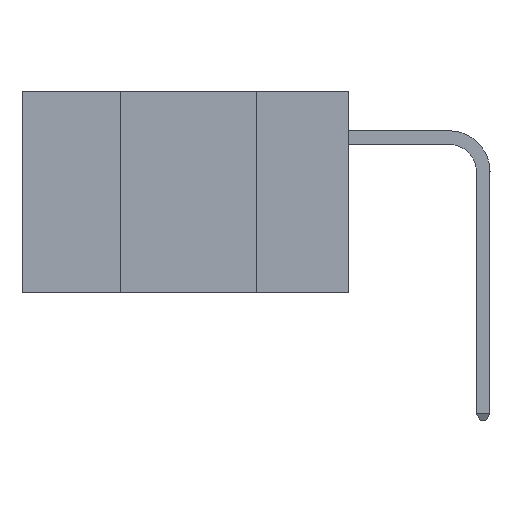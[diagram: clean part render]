
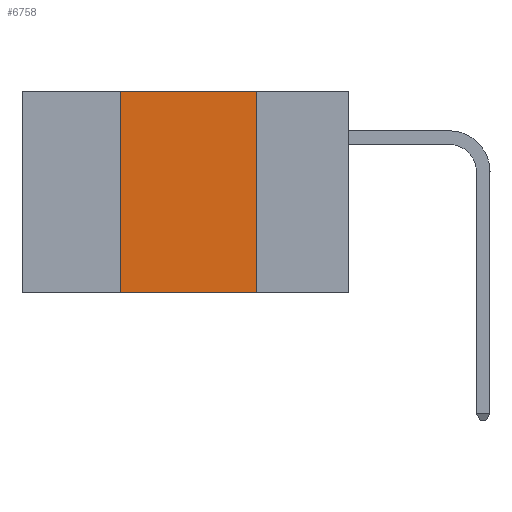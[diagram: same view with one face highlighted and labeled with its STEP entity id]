
A CAD part, left-side view. The second image highlights one B-rep face of the part: STEP entity #6758.
In plain terms, the highlighted planar face has unit normal (-1, 0, 0).
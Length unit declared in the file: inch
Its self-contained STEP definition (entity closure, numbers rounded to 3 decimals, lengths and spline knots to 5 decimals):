
#599 = DIRECTION ( 'NONE',  ( 1., 0., 0. ) ) ;
#921 = CARTESIAN_POINT ( 'NONE',  ( 0., 0.17, -0.37 ) ) ;
#3271 = ORIENTED_EDGE ( 'NONE', *, *, #20356, .F. ) ;
#4081 = DIRECTION ( 'NONE',  ( 0., -1., 0. ) ) ;
#4486 = CARTESIAN_POINT ( 'NONE',  ( 0., 0.17, 0. ) ) ;
#4714 = CARTESIAN_POINT ( 'NONE',  ( 0., 0.6, 0. ) ) ;
#6479 = EDGE_CURVE ( 'NONE', #21021, #20581, #16606, .T. ) ;
#6677 = CARTESIAN_POINT ( 'NONE',  ( 0., 0.42, 0. ) ) ;
#6758 = ADVANCED_FACE ( 'NONE', ( #10083 ), #6932, .F. ) ;
#6932 = PLANE ( 'NONE',  #14544 ) ;
#7320 = VECTOR ( 'NONE', #18434, 39.37008 ) ;
#8654 = CARTESIAN_POINT ( 'NONE',  ( 0., 0.6, 0. ) ) ;
#8744 = ORIENTED_EDGE ( 'NONE', *, *, #20480, .T. ) ;
#10083 = FACE_OUTER_BOUND ( 'NONE', #13795, .T. ) ;
#10695 = ORIENTED_EDGE ( 'NONE', *, *, #19570, .F. ) ;
#10784 = CARTESIAN_POINT ( 'NONE',  ( 0., 0.17, 0. ) ) ;
#11531 = VERTEX_POINT ( 'NONE', #6677 ) ;
#12270 = DIRECTION ( 'NONE',  ( 0., 0., -1. ) ) ;
#12802 = VERTEX_POINT ( 'NONE', #17006 ) ;
#12865 = CARTESIAN_POINT ( 'NONE',  ( 0., 0.6, -0.37 ) ) ;
#13220 = LINE ( 'NONE', #12865, #15654 ) ;
#13795 = EDGE_LOOP ( 'NONE', ( #14276, #10695, #3271, #8744 ) ) ;
#14276 = ORIENTED_EDGE ( 'NONE', *, *, #6479, .F. ) ;
#14324 = LINE ( 'NONE', #20907, #18294 ) ;
#14544 = AXIS2_PLACEMENT_3D ( 'NONE', #8654, #599, #12270 ) ;
#15654 = VECTOR ( 'NONE', #4081, 39.37008 ) ;
#15757 = DIRECTION ( 'NONE',  ( 0., 0., 1. ) ) ;
#16606 = LINE ( 'NONE', #4486, #7320 ) ;
#17006 = CARTESIAN_POINT ( 'NONE',  ( 0., 0.42, -0.37 ) ) ;
#18294 = VECTOR ( 'NONE', #15757, 39.37008 ) ;
#18434 = DIRECTION ( 'NONE',  ( 0., 0., -1. ) ) ;
#19570 = EDGE_CURVE ( 'NONE', #11531, #21021, #21285, .T. ) ;
#20356 = EDGE_CURVE ( 'NONE', #12802, #11531, #14324, .T. ) ;
#20480 = EDGE_CURVE ( 'NONE', #12802, #20581, #13220, .T. ) ;
#20581 = VERTEX_POINT ( 'NONE', #921 ) ;
#20764 = VECTOR ( 'NONE', #22137, 39.37008 ) ;
#20907 = CARTESIAN_POINT ( 'NONE',  ( 0., 0.42, 0. ) ) ;
#21021 = VERTEX_POINT ( 'NONE', #10784 ) ;
#21285 = LINE ( 'NONE', #4714, #20764 ) ;
#22137 = DIRECTION ( 'NONE',  ( 0., -1., 0. ) ) ;
